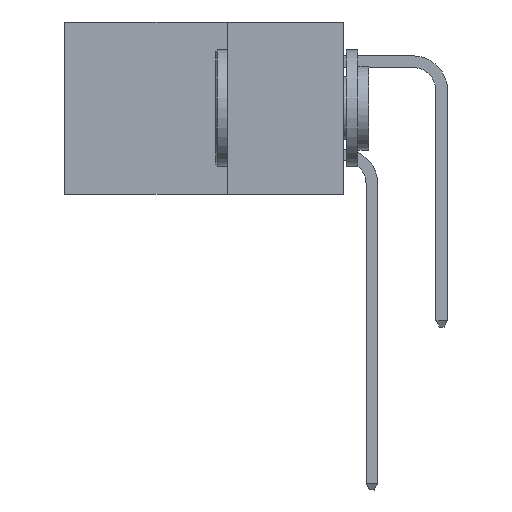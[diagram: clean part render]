
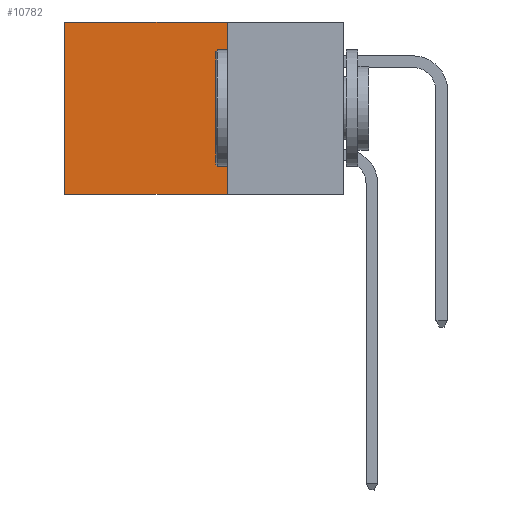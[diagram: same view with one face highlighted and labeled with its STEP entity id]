
A CAD part, left-side view. The second image highlights one B-rep face of the part: STEP entity #10782.
In plain terms, the highlighted planar face has unit normal (-1, 0, 0).
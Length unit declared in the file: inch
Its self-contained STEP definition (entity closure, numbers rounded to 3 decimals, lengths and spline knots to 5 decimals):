
#216 = VERTEX_POINT ( 'NONE', #3734 ) ;
#299 = CARTESIAN_POINT ( 'NONE',  ( 0.2615, 0.6, -0.37 ) ) ;
#1072 = LINE ( 'NONE', #5358, #3117 ) ;
#1449 = VECTOR ( 'NONE', #11279, 39.37008 ) ;
#1524 = EDGE_CURVE ( 'NONE', #216, #6631, #13585, .T. ) ;
#2522 = CARTESIAN_POINT ( 'NONE',  ( 0.2615, 0.6, 0. ) ) ;
#3117 = VECTOR ( 'NONE', #11849, 39.37008 ) ;
#3734 = CARTESIAN_POINT ( 'NONE',  ( 0.2615, 0.25, -0.37 ) ) ;
#3805 = PLANE ( 'NONE',  #5387 ) ;
#4415 = CARTESIAN_POINT ( 'NONE',  ( 0.2615, 0.25, -0.37 ) ) ;
#4889 = VECTOR ( 'NONE', #10046, 39.37008 ) ;
#4966 = CARTESIAN_POINT ( 'NONE',  ( 0.2615, 0.25, -0.37 ) ) ;
#5138 = ORIENTED_EDGE ( 'NONE', *, *, #8390, .T. ) ;
#5358 = CARTESIAN_POINT ( 'NONE',  ( 0.2615, 0.25, 0. ) ) ;
#5387 = AXIS2_PLACEMENT_3D ( 'NONE', #4966, #8182, #9309 ) ;
#5647 = LINE ( 'NONE', #299, #1449 ) ;
#6493 = ORIENTED_EDGE ( 'NONE', *, *, #1524, .F. ) ;
#6631 = VERTEX_POINT ( 'NONE', #7615 ) ;
#7615 = CARTESIAN_POINT ( 'NONE',  ( 0.2615, 0.6, -0.37 ) ) ;
#7972 = VERTEX_POINT ( 'NONE', #2522 ) ;
#8156 = ORIENTED_EDGE ( 'NONE', *, *, #8879, .F. ) ;
#8182 = DIRECTION ( 'NONE',  ( 1., 0., 0. ) ) ;
#8192 = CARTESIAN_POINT ( 'NONE',  ( 0.2615, 0.25, -0.37 ) ) ;
#8390 = EDGE_CURVE ( 'NONE', #7972, #6631, #5647, .T. ) ;
#8545 = VERTEX_POINT ( 'NONE', #9271 ) ;
#8879 = EDGE_CURVE ( 'NONE', #8545, #216, #12184, .T. ) ;
#8933 = VECTOR ( 'NONE', #11609, 39.37008 ) ;
#9072 = ORIENTED_EDGE ( 'NONE', *, *, #12059, .T. ) ;
#9271 = CARTESIAN_POINT ( 'NONE',  ( 0.2615, 0.25, 0. ) ) ;
#9309 = DIRECTION ( 'NONE',  ( 0., 0., -1. ) ) ;
#9411 = EDGE_LOOP ( 'NONE', ( #5138, #6493, #8156, #9072 ) ) ;
#10046 = DIRECTION ( 'NONE',  ( 0., 0., -1. ) ) ;
#10782 = ADVANCED_FACE ( 'NONE', ( #13788 ), #3805, .F. ) ;
#11279 = DIRECTION ( 'NONE',  ( 0., 0., -1. ) ) ;
#11609 = DIRECTION ( 'NONE',  ( 0., 1., 0. ) ) ;
#11849 = DIRECTION ( 'NONE',  ( 0., 1., 0. ) ) ;
#12059 = EDGE_CURVE ( 'NONE', #8545, #7972, #1072, .T. ) ;
#12184 = LINE ( 'NONE', #4415, #4889 ) ;
#13585 = LINE ( 'NONE', #8192, #8933 ) ;
#13788 = FACE_OUTER_BOUND ( 'NONE', #9411, .T. ) ;
